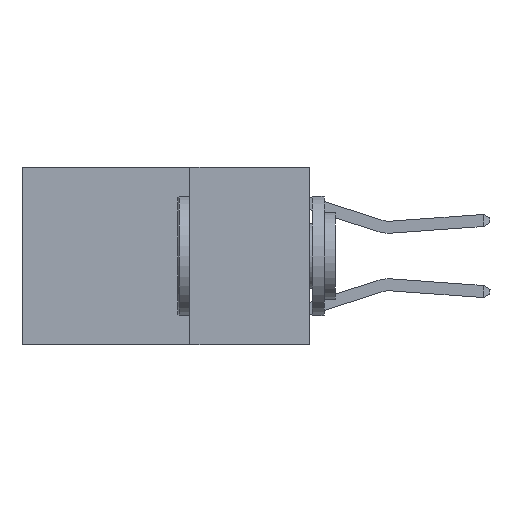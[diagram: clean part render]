
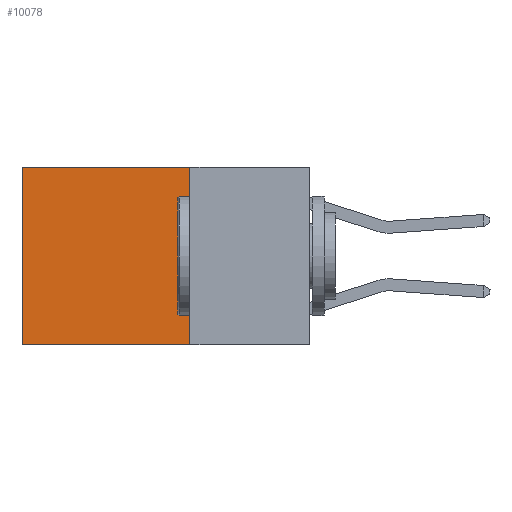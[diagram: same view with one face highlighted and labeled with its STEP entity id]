
A CAD part, left-side view. The second image highlights one B-rep face of the part: STEP entity #10078.
In plain terms, the highlighted planar face has unit normal (-1, 0, 0).
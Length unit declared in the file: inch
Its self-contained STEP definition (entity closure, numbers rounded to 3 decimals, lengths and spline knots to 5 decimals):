
#51 = ORIENTED_EDGE ( 'NONE', *, *, #525, .F. ) ;
#525 = EDGE_CURVE ( 'NONE', #4166, #25361, #21483, .T. ) ;
#1067 = PLANE ( 'NONE',  #30156 ) ;
#2735 = CARTESIAN_POINT ( 'NONE',  ( 0.2625, 0.25, 0. ) ) ;
#3048 = CARTESIAN_POINT ( 'NONE',  ( 0.2625, 0.6, -0.37 ) ) ;
#3648 = LINE ( 'NONE', #32002, #17062 ) ;
#4166 = VERTEX_POINT ( 'NONE', #8962 ) ;
#5369 = VERTEX_POINT ( 'NONE', #3048 ) ;
#5803 = ORIENTED_EDGE ( 'NONE', *, *, #7692, .T. ) ;
#6339 = EDGE_LOOP ( 'NONE', ( #15879, #27714, #51, #5803 ) ) ;
#7020 = LINE ( 'NONE', #2735, #26199 ) ;
#7692 = EDGE_CURVE ( 'NONE', #4166, #20643, #7020, .T. ) ;
#7947 = CARTESIAN_POINT ( 'NONE',  ( 0.2625, 0.25, 0. ) ) ;
#8380 = DIRECTION ( 'NONE',  ( 0., 0., -1. ) ) ;
#8679 = DIRECTION ( 'NONE',  ( 1., 0., 0. ) ) ;
#8962 = CARTESIAN_POINT ( 'NONE',  ( 0.2625, 0.25, 0. ) ) ;
#10078 = ADVANCED_FACE ( 'NONE', ( #11201 ), #1067, .F. ) ;
#10495 = CARTESIAN_POINT ( 'NONE',  ( 0.2625, 0.6, 0. ) ) ;
#11201 = FACE_OUTER_BOUND ( 'NONE', #6339, .T. ) ;
#12829 = DIRECTION ( 'NONE',  ( 0., 1., 0. ) ) ;
#14626 = VECTOR ( 'NONE', #26132, 39.37008 ) ;
#15753 = CARTESIAN_POINT ( 'NONE',  ( 0.2625, 0.25, -0.37 ) ) ;
#15879 = ORIENTED_EDGE ( 'NONE', *, *, #22210, .T. ) ;
#17062 = VECTOR ( 'NONE', #17203, 39.37008 ) ;
#17203 = DIRECTION ( 'NONE',  ( 0., 1., 0. ) ) ;
#20643 = VERTEX_POINT ( 'NONE', #10495 ) ;
#21483 = LINE ( 'NONE', #7947, #27289 ) ;
#22210 = EDGE_CURVE ( 'NONE', #20643, #5369, #22831, .T. ) ;
#22831 = LINE ( 'NONE', #23661, #14626 ) ;
#23661 = CARTESIAN_POINT ( 'NONE',  ( 0.2625, 0.6, 0. ) ) ;
#23702 = CARTESIAN_POINT ( 'NONE',  ( 0.2625, 0.25, 0. ) ) ;
#25361 = VERTEX_POINT ( 'NONE', #15753 ) ;
#26132 = DIRECTION ( 'NONE',  ( 0., 0., -1. ) ) ;
#26175 = DIRECTION ( 'NONE',  ( 0., 0., -1. ) ) ;
#26199 = VECTOR ( 'NONE', #12829, 39.37008 ) ;
#26873 = EDGE_CURVE ( 'NONE', #25361, #5369, #3648, .T. ) ;
#27289 = VECTOR ( 'NONE', #8380, 39.37008 ) ;
#27714 = ORIENTED_EDGE ( 'NONE', *, *, #26873, .F. ) ;
#30156 = AXIS2_PLACEMENT_3D ( 'NONE', #23702, #8679, #26175 ) ;
#32002 = CARTESIAN_POINT ( 'NONE',  ( 0.2625, 0.25, -0.37 ) ) ;
